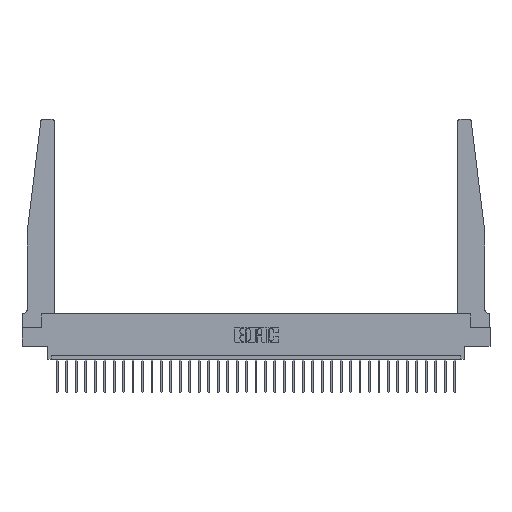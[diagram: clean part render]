
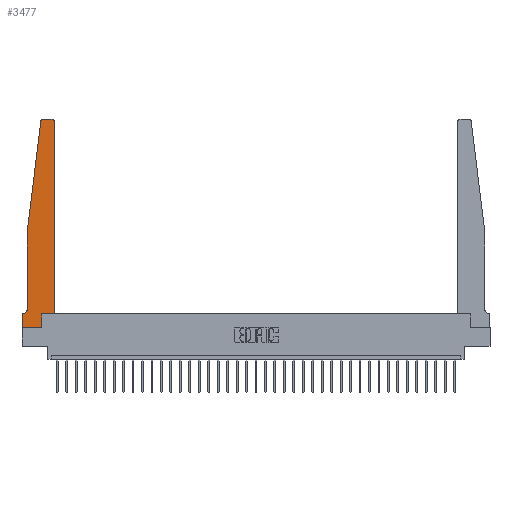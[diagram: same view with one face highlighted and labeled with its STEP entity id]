
A CAD part, top view. The second image highlights one B-rep face of the part: STEP entity #3477.
In plain terms, the highlighted planar face has unit normal (0, 0, 1).
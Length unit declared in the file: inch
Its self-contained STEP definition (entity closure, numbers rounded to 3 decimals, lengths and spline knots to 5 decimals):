
#116 = CARTESIAN_POINT ( 'NONE',  ( 0.065, 1.25, 0.37 ) ) ;
#373 = DIRECTION ( 'NONE',  ( 1., 0., 0. ) ) ;
#549 = VERTEX_POINT ( 'NONE', #23754 ) ;
#761 = VERTEX_POINT ( 'NONE', #18063 ) ;
#1065 = DIRECTION ( 'NONE',  ( 0., -1., 0. ) ) ;
#1881 = CARTESIAN_POINT ( 'NONE',  ( 0., 0., 0.37 ) ) ;
#2028 = DIRECTION ( 'NONE',  ( 1., 0., 0. ) ) ;
#2100 = VECTOR ( 'NONE', #28206, 39.37008 ) ;
#2297 = CARTESIAN_POINT ( 'NONE',  ( 0., 0.1875, 0.37 ) ) ;
#2315 = LINE ( 'NONE', #21404, #19445 ) ;
#2611 = CARTESIAN_POINT ( 'NONE',  ( 0.395, 2.72, 0.37 ) ) ;
#2716 = DIRECTION ( 'NONE',  ( 0., 0., 1. ) ) ;
#2898 = EDGE_CURVE ( 'NONE', #4724, #20860, #10673, .T. ) ;
#3274 = VECTOR ( 'NONE', #22644, 39.37008 ) ;
#3477 = ADVANCED_FACE ( 'NONE', ( #5734 ), #14173, .T. ) ;
#3589 = EDGE_CURVE ( 'NONE', #549, #21574, #9113, .T. ) ;
#3999 = EDGE_CURVE ( 'NONE', #26677, #761, #20334, .T. ) ;
#4035 = LINE ( 'NONE', #19459, #3274 ) ;
#4075 = ORIENTED_EDGE ( 'NONE', *, *, #18444, .T. ) ;
#4189 = VECTOR ( 'NONE', #1065, 39.37008 ) ;
#4246 = VECTOR ( 'NONE', #17151, 39.37008 ) ;
#4504 = ORIENTED_EDGE ( 'NONE', *, *, #21098, .T. ) ;
#4558 = VERTEX_POINT ( 'NONE', #21480 ) ;
#4628 = VERTEX_POINT ( 'NONE', #18845 ) ;
#4724 = VERTEX_POINT ( 'NONE', #15646 ) ;
#5734 = FACE_OUTER_BOUND ( 'NONE', #14927, .T. ) ;
#5866 = VECTOR ( 'NONE', #21555, 39.37008 ) ;
#5967 = ORIENTED_EDGE ( 'NONE', *, *, #15556, .T. ) ;
#6153 = ORIENTED_EDGE ( 'NONE', *, *, #30161, .T. ) ;
#6196 = AXIS2_PLACEMENT_3D ( 'NONE', #28828, #9436, #2028 ) ;
#6277 = DIRECTION ( 'NONE',  ( 0., 0., -1. ) ) ;
#6682 = CARTESIAN_POINT ( 'NONE',  ( 0.425, 0.18, 0.37 ) ) ;
#6934 = ORIENTED_EDGE ( 'NONE', *, *, #3999, .T. ) ;
#7500 = CARTESIAN_POINT ( 'NONE',  ( 0.065, 1.25, 0.37 ) ) ;
#7548 = CARTESIAN_POINT ( 'NONE',  ( 0.065, 0.2375, 0.37 ) ) ;
#7916 = EDGE_CURVE ( 'NONE', #21574, #11490, #18056, .T. ) ;
#8065 = CARTESIAN_POINT ( 'NONE',  ( 0., 0., 0.37 ) ) ;
#8465 = AXIS2_PLACEMENT_3D ( 'NONE', #2611, #2716, #373 ) ;
#9113 = CIRCLE ( 'NONE', #8465, 0.03 ) ;
#9247 = DIRECTION ( 'NONE',  ( -1., 0., 0. ) ) ;
#9309 = LINE ( 'NONE', #23310, #2100 ) ;
#9436 = DIRECTION ( 'NONE',  ( 0., 0., 1. ) ) ;
#9627 = ORIENTED_EDGE ( 'NONE', *, *, #24100, .T. ) ;
#9666 = ORIENTED_EDGE ( 'NONE', *, *, #11930, .T. ) ;
#10667 = AXIS2_PLACEMENT_3D ( 'NONE', #25892, #6277, #28340 ) ;
#10673 = LINE ( 'NONE', #116, #4246 ) ;
#11069 = ORIENTED_EDGE ( 'NONE', *, *, #23168, .T. ) ;
#11388 = CIRCLE ( 'NONE', #6196, 0.03 ) ;
#11490 = VERTEX_POINT ( 'NONE', #28650 ) ;
#11605 = CARTESIAN_POINT ( 'NONE',  ( 0.065, 1.25, 0.37 ) ) ;
#11930 = EDGE_CURVE ( 'NONE', #27428, #4558, #9309, .T. ) ;
#11997 = VERTEX_POINT ( 'NONE', #15488 ) ;
#12220 = VERTEX_POINT ( 'NONE', #1881 ) ;
#13949 = ORIENTED_EDGE ( 'NONE', *, *, #2898, .T. ) ;
#14173 = PLANE ( 'NONE',  #22743 ) ;
#14927 = EDGE_LOOP ( 'NONE', ( #19094, #9627, #13949, #11069, #6934, #4075, #5967, #25461, #4504, #9666, #6153, #18744 ) ) ;
#15026 = DIRECTION ( 'NONE',  ( 0., -1., 0. ) ) ;
#15147 = CARTESIAN_POINT ( 'NONE',  ( 0., 0., 0.37 ) ) ;
#15488 = CARTESIAN_POINT ( 'NONE',  ( 0., 0.1875, 0.37 ) ) ;
#15556 = EDGE_CURVE ( 'NONE', #11997, #12220, #26266, .T. ) ;
#15646 = CARTESIAN_POINT ( 'NONE',  ( 0.24675, 2.72367, 0.37 ) ) ;
#17151 = DIRECTION ( 'NONE',  ( -0.122, -0.992, 0. ) ) ;
#17513 = CARTESIAN_POINT ( 'NONE',  ( 0.2605, 0.18, 0.37 ) ) ;
#18056 = LINE ( 'NONE', #21343, #5866 ) ;
#18063 = CARTESIAN_POINT ( 'NONE',  ( 0.015, 0.1875, 0.37 ) ) ;
#18444 = EDGE_CURVE ( 'NONE', #761, #11997, #2315, .T. ) ;
#18542 = VECTOR ( 'NONE', #27425, 39.37008 ) ;
#18724 = DIRECTION ( 'NONE',  ( 0., 1., 0. ) ) ;
#18744 = ORIENTED_EDGE ( 'NONE', *, *, #3589, .T. ) ;
#18845 = CARTESIAN_POINT ( 'NONE',  ( 0.2605, 0., 0.37 ) ) ;
#19094 = ORIENTED_EDGE ( 'NONE', *, *, #7916, .T. ) ;
#19323 = DIRECTION ( 'NONE',  ( 0., 0., 1. ) ) ;
#19362 = VECTOR ( 'NONE', #18724, 39.37008 ) ;
#19445 = VECTOR ( 'NONE', #9247, 39.37008 ) ;
#19459 = CARTESIAN_POINT ( 'NONE',  ( 0.2605, 0.18, 0.37 ) ) ;
#20017 = EDGE_CURVE ( 'NONE', #12220, #4628, #23509, .T. ) ;
#20334 = CIRCLE ( 'NONE', #10667, 0.05 ) ;
#20635 = VECTOR ( 'NONE', #15026, 39.37008 ) ;
#20860 = VERTEX_POINT ( 'NONE', #11605 ) ;
#21098 = EDGE_CURVE ( 'NONE', #4628, #27428, #4035, .T. ) ;
#21343 = CARTESIAN_POINT ( 'NONE',  ( 0.25, 2.75, 0.37 ) ) ;
#21404 = CARTESIAN_POINT ( 'NONE',  ( 0.065, 0.1875, 0.37 ) ) ;
#21480 = CARTESIAN_POINT ( 'NONE',  ( 0.425, 0.18, 0.37 ) ) ;
#21555 = DIRECTION ( 'NONE',  ( -1., 0., 0. ) ) ;
#21574 = VERTEX_POINT ( 'NONE', #22454 ) ;
#22454 = CARTESIAN_POINT ( 'NONE',  ( 0.395, 2.75, 0.37 ) ) ;
#22644 = DIRECTION ( 'NONE',  ( 0., 1., 0. ) ) ;
#22743 = AXIS2_PLACEMENT_3D ( 'NONE', #2297, #19323, #26570 ) ;
#23168 = EDGE_CURVE ( 'NONE', #20860, #26677, #27889, .T. ) ;
#23310 = CARTESIAN_POINT ( 'NONE',  ( 0.425, 0.18, 0.37 ) ) ;
#23509 = LINE ( 'NONE', #15147, #18542 ) ;
#23754 = CARTESIAN_POINT ( 'NONE',  ( 0.425, 2.72, 0.37 ) ) ;
#24100 = EDGE_CURVE ( 'NONE', #11490, #4724, #11388, .T. ) ;
#25054 = LINE ( 'NONE', #6682, #19362 ) ;
#25461 = ORIENTED_EDGE ( 'NONE', *, *, #20017, .T. ) ;
#25892 = CARTESIAN_POINT ( 'NONE',  ( 0.015, 0.2375, 0.37 ) ) ;
#26266 = LINE ( 'NONE', #8065, #4189 ) ;
#26570 = DIRECTION ( 'NONE',  ( 1., 0., 0. ) ) ;
#26677 = VERTEX_POINT ( 'NONE', #7548 ) ;
#27425 = DIRECTION ( 'NONE',  ( 1., 0., 0. ) ) ;
#27428 = VERTEX_POINT ( 'NONE', #17513 ) ;
#27889 = LINE ( 'NONE', #7500, #20635 ) ;
#28206 = DIRECTION ( 'NONE',  ( 1., 0., 0. ) ) ;
#28340 = DIRECTION ( 'NONE',  ( -1., 0., 0. ) ) ;
#28650 = CARTESIAN_POINT ( 'NONE',  ( 0.27653, 2.75, 0.37 ) ) ;
#28828 = CARTESIAN_POINT ( 'NONE',  ( 0.27653, 2.72, 0.37 ) ) ;
#30161 = EDGE_CURVE ( 'NONE', #4558, #549, #25054, .T. ) ;
